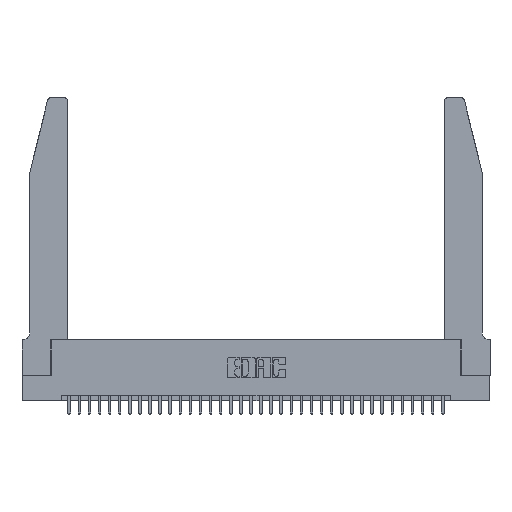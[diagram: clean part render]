
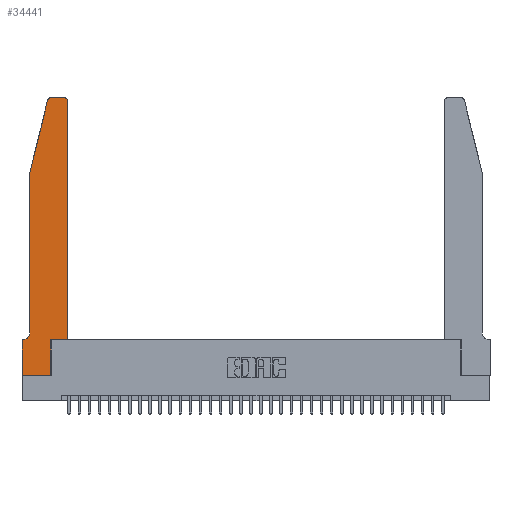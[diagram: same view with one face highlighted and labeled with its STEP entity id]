
A CAD part, top view. The second image highlights one B-rep face of the part: STEP entity #34441.
In plain terms, the highlighted planar face has unit normal (0, 0, 1).
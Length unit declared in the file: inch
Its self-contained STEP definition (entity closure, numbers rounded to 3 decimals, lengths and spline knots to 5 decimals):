
#100 = VECTOR ( 'NONE', #7421, 39.37008 ) ;
#112 = VERTEX_POINT ( 'NONE', #4720 ) ;
#380 = ORIENTED_EDGE ( 'NONE', *, *, #11434, .T. ) ;
#556 = ORIENTED_EDGE ( 'NONE', *, *, #6562, .T. ) ;
#828 = CARTESIAN_POINT ( 'NONE',  ( 0.284, 2.75, 0.37 ) ) ;
#939 = CARTESIAN_POINT ( 'NONE',  ( 0.0755, 0.35, 0.37 ) ) ;
#2152 = DIRECTION ( 'NONE',  ( 0., 0., -1. ) ) ;
#2173 = ORIENTED_EDGE ( 'NONE', *, *, #12126, .T. ) ;
#2344 = VECTOR ( 'NONE', #17745, 39.37008 ) ;
#2538 = LINE ( 'NONE', #7814, #9039 ) ;
#3340 = VERTEX_POINT ( 'NONE', #19382 ) ;
#3539 = EDGE_CURVE ( 'NONE', #10422, #12906, #23162, .T. ) ;
#4720 = CARTESIAN_POINT ( 'NONE',  ( 0.0055, 0.35, 0.37 ) ) ;
#4885 = CARTESIAN_POINT ( 'NONE',  ( 0., 0.35, 0.37 ) ) ;
#5128 = CIRCLE ( 'NONE', #32354, 0.03 ) ;
#5184 = AXIS2_PLACEMENT_3D ( 'NONE', #4885, #10457, #29358 ) ;
#5368 = CARTESIAN_POINT ( 'NONE',  ( 0.2865, 0.35, 0.37 ) ) ;
#6389 = CARTESIAN_POINT ( 'NONE',  ( 0.4505, 0.35, 0.37 ) ) ;
#6562 = EDGE_CURVE ( 'NONE', #15016, #16206, #32977, .T. ) ;
#7421 = DIRECTION ( 'NONE',  ( 0., -1., 0. ) ) ;
#7733 = DIRECTION ( 'NONE',  ( 1., 0., 0. ) ) ;
#7750 = ORIENTED_EDGE ( 'NONE', *, *, #3539, .T. ) ;
#7814 = CARTESIAN_POINT ( 'NONE',  ( 0.0755, 2., 0.37 ) ) ;
#8317 = VECTOR ( 'NONE', #22852, 39.37008 ) ;
#8359 = DIRECTION ( 'NONE',  ( 0., 0., 1. ) ) ;
#8465 = CARTESIAN_POINT ( 'NONE',  ( 0.2605, 2.75, 0.37 ) ) ;
#8743 = CARTESIAN_POINT ( 'NONE',  ( 0., 0., 0.37 ) ) ;
#9039 = VECTOR ( 'NONE', #10591, 39.37008 ) ;
#9076 = ORIENTED_EDGE ( 'NONE', *, *, #14374, .T. ) ;
#9523 = CARTESIAN_POINT ( 'NONE',  ( 0., 0., 0.37 ) ) ;
#10105 = DIRECTION ( 'NONE',  ( 0., 1., 0. ) ) ;
#10422 = VERTEX_POINT ( 'NONE', #16740 ) ;
#10457 = DIRECTION ( 'NONE',  ( 0., 0., 1. ) ) ;
#10591 = DIRECTION ( 'NONE',  ( -0.239, -0.971, 0. ) ) ;
#10947 = DIRECTION ( 'NONE',  ( 0., 0., 1. ) ) ;
#11203 = ORIENTED_EDGE ( 'NONE', *, *, #34170, .T. ) ;
#11434 = EDGE_CURVE ( 'NONE', #3340, #15016, #5128, .T. ) ;
#11490 = CARTESIAN_POINT ( 'NONE',  ( 0.0755, 2., 0.37 ) ) ;
#11862 = CIRCLE ( 'NONE', #28731, 0.03 ) ;
#12126 = EDGE_CURVE ( 'NONE', #17332, #10422, #12828, .T. ) ;
#12326 = VECTOR ( 'NONE', #27426, 39.37008 ) ;
#12580 = CARTESIAN_POINT ( 'NONE',  ( 0., 0.35, 0.37 ) ) ;
#12722 = EDGE_CURVE ( 'NONE', #29156, #3340, #18344, .T. ) ;
#12828 = LINE ( 'NONE', #24030, #35124 ) ;
#12906 = VERTEX_POINT ( 'NONE', #5368 ) ;
#13511 = CARTESIAN_POINT ( 'NONE',  ( 0.25487, 2.72718, 0.37 ) ) ;
#14374 = EDGE_CURVE ( 'NONE', #32593, #17332, #24964, .T. ) ;
#14568 = FACE_OUTER_BOUND ( 'NONE', #29494, .T. ) ;
#14589 = ORIENTED_EDGE ( 'NONE', *, *, #23887, .T. ) ;
#14617 = DIRECTION ( 'NONE',  ( 1., 0., 0. ) ) ;
#15016 = VERTEX_POINT ( 'NONE', #26214 ) ;
#15253 = VERTEX_POINT ( 'NONE', #13511 ) ;
#15939 = VECTOR ( 'NONE', #31340, 39.37008 ) ;
#16082 = ORIENTED_EDGE ( 'NONE', *, *, #19729, .T. ) ;
#16206 = VERTEX_POINT ( 'NONE', #828 ) ;
#16435 = LINE ( 'NONE', #939, #8317 ) ;
#16740 = CARTESIAN_POINT ( 'NONE',  ( 0.2865, 0., 0.37 ) ) ;
#16759 = VECTOR ( 'NONE', #14617, 39.37008 ) ;
#17099 = CARTESIAN_POINT ( 'NONE',  ( 0.0755, 0.42, 0.37 ) ) ;
#17332 = VERTEX_POINT ( 'NONE', #8743 ) ;
#17611 = LINE ( 'NONE', #6389, #16759 ) ;
#17745 = DIRECTION ( 'NONE',  ( 0., -1., 0. ) ) ;
#18344 = LINE ( 'NONE', #31699, #23828 ) ;
#18580 = CARTESIAN_POINT ( 'NONE',  ( 0.0055, 0.42, 0.37 ) ) ;
#19382 = CARTESIAN_POINT ( 'NONE',  ( 0.4505, 2.72, 0.37 ) ) ;
#19635 = AXIS2_PLACEMENT_3D ( 'NONE', #18580, #2152, #21292 ) ;
#19729 = EDGE_CURVE ( 'NONE', #16206, #15253, #11862, .T. ) ;
#21292 = DIRECTION ( 'NONE',  ( -1., 0., 0. ) ) ;
#22852 = DIRECTION ( 'NONE',  ( -1., 0., 0. ) ) ;
#23162 = LINE ( 'NONE', #23282, #15939 ) ;
#23282 = CARTESIAN_POINT ( 'NONE',  ( 0.2865, 0.35, 0.37 ) ) ;
#23731 = CARTESIAN_POINT ( 'NONE',  ( 0.0755, 2., 0.37 ) ) ;
#23781 = ORIENTED_EDGE ( 'NONE', *, *, #12722, .T. ) ;
#23828 = VECTOR ( 'NONE', #10105, 39.37008 ) ;
#23887 = EDGE_CURVE ( 'NONE', #15253, #27393, #2538, .T. ) ;
#24030 = CARTESIAN_POINT ( 'NONE',  ( 0., 0., 0.37 ) ) ;
#24632 = CARTESIAN_POINT ( 'NONE',  ( 0.284, 2.72, 0.37 ) ) ;
#24964 = LINE ( 'NONE', #9523, #2344 ) ;
#26214 = CARTESIAN_POINT ( 'NONE',  ( 0.4205, 2.75, 0.37 ) ) ;
#26438 = EDGE_CURVE ( 'NONE', #31869, #112, #27070, .T. ) ;
#26702 = PLANE ( 'NONE',  #5184 ) ;
#27070 = CIRCLE ( 'NONE', #19635, 0.07 ) ;
#27071 = EDGE_CURVE ( 'NONE', #27393, #31869, #34494, .T. ) ;
#27170 = CARTESIAN_POINT ( 'NONE',  ( 0.4205, 2.72, 0.37 ) ) ;
#27327 = DIRECTION ( 'NONE',  ( 1., 0., 0. ) ) ;
#27393 = VERTEX_POINT ( 'NONE', #11490 ) ;
#27426 = DIRECTION ( 'NONE',  ( -1., 0., 0. ) ) ;
#28034 = ORIENTED_EDGE ( 'NONE', *, *, #27071, .T. ) ;
#28107 = EDGE_CURVE ( 'NONE', #112, #32593, #16435, .T. ) ;
#28731 = AXIS2_PLACEMENT_3D ( 'NONE', #24632, #8359, #27327 ) ;
#29156 = VERTEX_POINT ( 'NONE', #29689 ) ;
#29358 = DIRECTION ( 'NONE',  ( 1., 0., 0. ) ) ;
#29453 = ORIENTED_EDGE ( 'NONE', *, *, #26438, .T. ) ;
#29494 = EDGE_LOOP ( 'NONE', ( #556, #16082, #14589, #28034, #29453, #30447, #9076, #2173, #7750, #11203, #23781, #380 ) ) ;
#29689 = CARTESIAN_POINT ( 'NONE',  ( 0.4505, 0.35, 0.37 ) ) ;
#29845 = DIRECTION ( 'NONE',  ( 1., 0., 0. ) ) ;
#30447 = ORIENTED_EDGE ( 'NONE', *, *, #28107, .T. ) ;
#31340 = DIRECTION ( 'NONE',  ( 0., 1., 0. ) ) ;
#31699 = CARTESIAN_POINT ( 'NONE',  ( 0.4505, 0.35, 0.37 ) ) ;
#31869 = VERTEX_POINT ( 'NONE', #17099 ) ;
#32354 = AXIS2_PLACEMENT_3D ( 'NONE', #27170, #10947, #29845 ) ;
#32593 = VERTEX_POINT ( 'NONE', #12580 ) ;
#32977 = LINE ( 'NONE', #8465, #12326 ) ;
#34170 = EDGE_CURVE ( 'NONE', #12906, #29156, #17611, .T. ) ;
#34441 = ADVANCED_FACE ( 'NONE', ( #14568 ), #26702, .T. ) ;
#34494 = LINE ( 'NONE', #23731, #100 ) ;
#35124 = VECTOR ( 'NONE', #7733, 39.37008 ) ;
